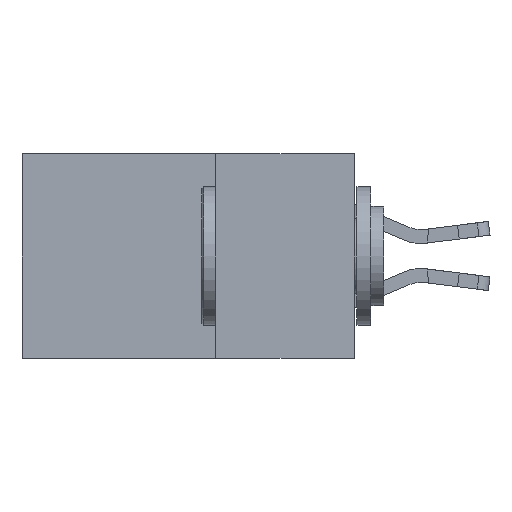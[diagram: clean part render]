
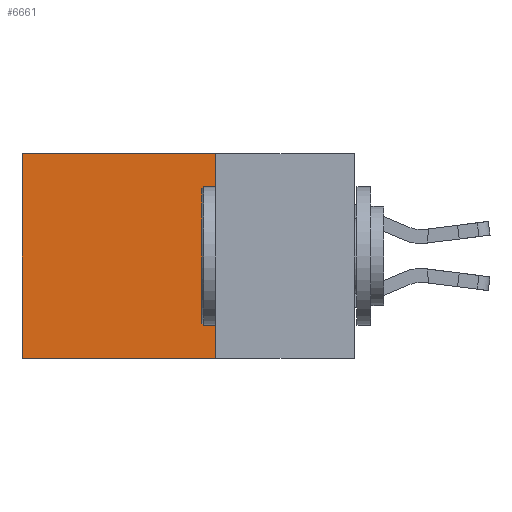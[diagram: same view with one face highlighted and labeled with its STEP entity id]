
A CAD part, left-side view. The second image highlights one B-rep face of the part: STEP entity #6661.
In plain terms, the highlighted planar face has unit normal (-1, 0, 0).
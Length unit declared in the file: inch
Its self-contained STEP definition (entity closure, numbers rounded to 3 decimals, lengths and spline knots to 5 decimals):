
#39 = CARTESIAN_POINT ( 'NONE',  ( 0.2615, 0.6, 0. ) ) ;
#512 = CARTESIAN_POINT ( 'NONE',  ( 0.2615, 0.25, -0.37 ) ) ;
#1434 = EDGE_CURVE ( 'NONE', #5170, #8198, #17786, .T. ) ;
#2069 = CARTESIAN_POINT ( 'NONE',  ( 0.2615, 0.6, -0.37 ) ) ;
#2175 = CARTESIAN_POINT ( 'NONE',  ( 0.2615, 0.25, -0.37 ) ) ;
#2742 = LINE ( 'NONE', #6491, #9854 ) ;
#2831 = CARTESIAN_POINT ( 'NONE',  ( 0.2615, 0.6, -0.37 ) ) ;
#2944 = ORIENTED_EDGE ( 'NONE', *, *, #21674, .F. ) ;
#4709 = LINE ( 'NONE', #12130, #15255 ) ;
#5170 = VERTEX_POINT ( 'NONE', #39 ) ;
#6491 = CARTESIAN_POINT ( 'NONE',  ( 0.2615, 0.25, -0.37 ) ) ;
#6661 = ADVANCED_FACE ( 'NONE', ( #9491 ), #16917, .F. ) ;
#6908 = CARTESIAN_POINT ( 'NONE',  ( 0.2615, 0.25, -0.37 ) ) ;
#7836 = VECTOR ( 'NONE', #10604, 39.37008 ) ;
#8198 = VERTEX_POINT ( 'NONE', #2069 ) ;
#9491 = FACE_OUTER_BOUND ( 'NONE', #20205, .T. ) ;
#9854 = VECTOR ( 'NONE', #12100, 39.37008 ) ;
#10183 = CARTESIAN_POINT ( 'NONE',  ( 0.2615, 0.25, 0. ) ) ;
#10604 = DIRECTION ( 'NONE',  ( 0., 0., -1. ) ) ;
#12100 = DIRECTION ( 'NONE',  ( 0., 0., -1. ) ) ;
#12130 = CARTESIAN_POINT ( 'NONE',  ( 0.2615, 0.25, 0. ) ) ;
#13600 = ORIENTED_EDGE ( 'NONE', *, *, #20736, .F. ) ;
#15222 = VECTOR ( 'NONE', #21712, 39.37008 ) ;
#15255 = VECTOR ( 'NONE', #19523, 39.37008 ) ;
#15880 = ORIENTED_EDGE ( 'NONE', *, *, #16690, .T. ) ;
#16040 = LINE ( 'NONE', #6908, #15222 ) ;
#16416 = VERTEX_POINT ( 'NONE', #2175 ) ;
#16690 = EDGE_CURVE ( 'NONE', #17970, #5170, #4709, .T. ) ;
#16917 = PLANE ( 'NONE',  #19275 ) ;
#17786 = LINE ( 'NONE', #2831, #7836 ) ;
#17970 = VERTEX_POINT ( 'NONE', #10183 ) ;
#19275 = AXIS2_PLACEMENT_3D ( 'NONE', #512, #20436, #20558 ) ;
#19523 = DIRECTION ( 'NONE',  ( 0., 1., 0. ) ) ;
#20205 = EDGE_LOOP ( 'NONE', ( #20710, #13600, #2944, #15880 ) ) ;
#20436 = DIRECTION ( 'NONE',  ( 1., 0., 0. ) ) ;
#20558 = DIRECTION ( 'NONE',  ( 0., 0., -1. ) ) ;
#20710 = ORIENTED_EDGE ( 'NONE', *, *, #1434, .T. ) ;
#20736 = EDGE_CURVE ( 'NONE', #16416, #8198, #16040, .T. ) ;
#21674 = EDGE_CURVE ( 'NONE', #17970, #16416, #2742, .T. ) ;
#21712 = DIRECTION ( 'NONE',  ( 0., 1., 0. ) ) ;
